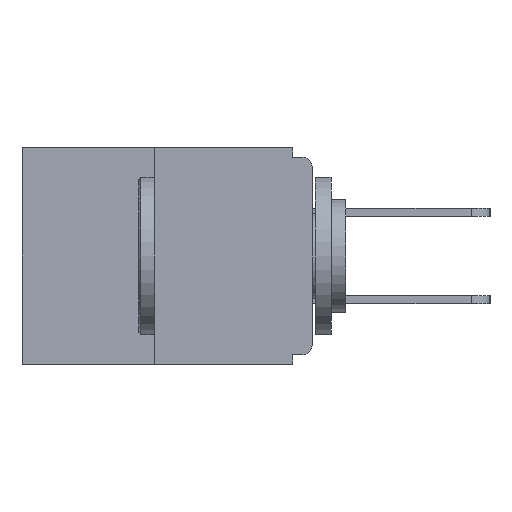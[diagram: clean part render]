
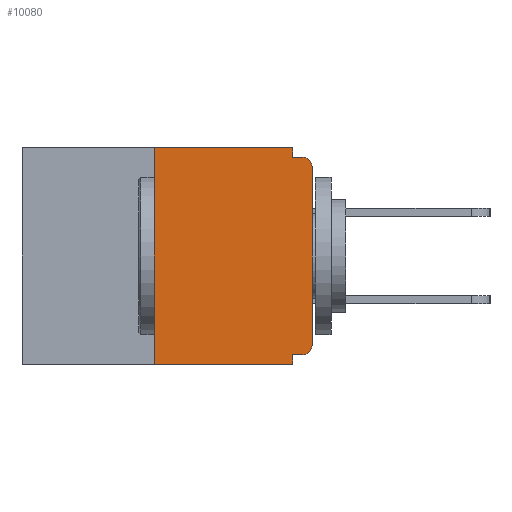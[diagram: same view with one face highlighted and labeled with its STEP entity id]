
A CAD part, left-side view. The second image highlights one B-rep face of the part: STEP entity #10080.
In plain terms, the highlighted planar face has unit normal (-1, 0, 0).
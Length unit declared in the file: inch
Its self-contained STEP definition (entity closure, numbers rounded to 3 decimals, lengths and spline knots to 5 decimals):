
#145 = ORIENTED_EDGE ( 'NONE', *, *, #12287, .T. ) ;
#869 = CARTESIAN_POINT ( 'NONE',  ( 0., 0., -0.03 ) ) ;
#907 = CARTESIAN_POINT ( 'NONE',  ( 0., 0.031, -0.328 ) ) ;
#1152 = CARTESIAN_POINT ( 'NONE',  ( 0., 0.015, -0.313 ) ) ;
#1493 = EDGE_CURVE ( 'NONE', #26048, #3067, #26186, .T. ) ;
#3067 = VERTEX_POINT ( 'NONE', #28551 ) ;
#3303 = ORIENTED_EDGE ( 'NONE', *, *, #7014, .F. ) ;
#3321 = VERTEX_POINT ( 'NONE', #26384 ) ;
#3494 = VERTEX_POINT ( 'NONE', #907 ) ;
#3663 = VECTOR ( 'NONE', #24541, 39.37008 ) ;
#3852 = AXIS2_PLACEMENT_3D ( 'NONE', #1152, #8369, #25537 ) ;
#4375 = CARTESIAN_POINT ( 'NONE',  ( 0., 0., -0.015 ) ) ;
#4817 = LINE ( 'NONE', #4375, #13469 ) ;
#5482 = CARTESIAN_POINT ( 'NONE',  ( 0., 0.46, -0.343 ) ) ;
#6423 = VERTEX_POINT ( 'NONE', #19023 ) ;
#6608 = ORIENTED_EDGE ( 'NONE', *, *, #12519, .F. ) ;
#6713 = VECTOR ( 'NONE', #14352, 39.37008 ) ;
#7014 = EDGE_CURVE ( 'NONE', #6423, #3494, #13935, .T. ) ;
#7239 = LINE ( 'NONE', #16847, #10235 ) ;
#7670 = DIRECTION ( 'NONE',  ( 1., 0., 0. ) ) ;
#8369 = DIRECTION ( 'NONE',  ( -1., 0., 0. ) ) ;
#8530 = LINE ( 'NONE', #5482, #3663 ) ;
#8600 = DIRECTION ( 'NONE',  ( 0., -1., 0. ) ) ;
#8676 = EDGE_CURVE ( 'NONE', #24810, #23961, #8530, .T. ) ;
#8923 = ORIENTED_EDGE ( 'NONE', *, *, #1493, .T. ) ;
#9445 = ORIENTED_EDGE ( 'NONE', *, *, #8676, .T. ) ;
#9480 = EDGE_CURVE ( 'NONE', #3494, #23961, #7239, .T. ) ;
#9860 = DIRECTION ( 'NONE',  ( 0., 0., -1. ) ) ;
#10080 = ADVANCED_FACE ( 'NONE', ( #20475 ), #29157, .F. ) ;
#10235 = VECTOR ( 'NONE', #21683, 39.37008 ) ;
#10701 = CARTESIAN_POINT ( 'NONE',  ( 0., 0., -0.313 ) ) ;
#11185 = EDGE_CURVE ( 'NONE', #29660, #11594, #11668, .T. ) ;
#11594 = VERTEX_POINT ( 'NONE', #20174 ) ;
#11668 = LINE ( 'NONE', #25041, #23734 ) ;
#12287 = EDGE_CURVE ( 'NONE', #6423, #23241, #21100, .T. ) ;
#12415 = CARTESIAN_POINT ( 'NONE',  ( 0., 0.46, 0. ) ) ;
#12519 = EDGE_CURVE ( 'NONE', #11594, #3321, #25159, .T. ) ;
#12708 = DIRECTION ( 'NONE',  ( -1., 0., 0. ) ) ;
#13469 = VECTOR ( 'NONE', #21218, 39.37008 ) ;
#13855 = EDGE_LOOP ( 'NONE', ( #15466, #15655, #9445, #22536, #3303, #145, #29830, #8923, #30356, #6608 ) ) ;
#13935 = LINE ( 'NONE', #28891, #27871 ) ;
#14167 = CARTESIAN_POINT ( 'NONE',  ( 0., 0.031, -0.343 ) ) ;
#14352 = DIRECTION ( 'NONE',  ( 0., 0., -1. ) ) ;
#15230 = DIRECTION ( 'NONE',  ( 0., 0., -1. ) ) ;
#15466 = ORIENTED_EDGE ( 'NONE', *, *, #11185, .F. ) ;
#15655 = ORIENTED_EDGE ( 'NONE', *, *, #23922, .F. ) ;
#15932 = CARTESIAN_POINT ( 'NONE',  ( 0., 0.25, 0. ) ) ;
#16706 = CARTESIAN_POINT ( 'NONE',  ( 0., 0.031, 0. ) ) ;
#16810 = DIRECTION ( 'NONE',  ( 0., 1., 0. ) ) ;
#16847 = CARTESIAN_POINT ( 'NONE',  ( 0., 0.031, -0.343 ) ) ;
#18273 = CARTESIAN_POINT ( 'NONE',  ( 0., 0.25, -0.343 ) ) ;
#19023 = CARTESIAN_POINT ( 'NONE',  ( 0., 0.015, -0.328 ) ) ;
#19800 = EDGE_CURVE ( 'NONE', #3321, #3067, #4817, .T. ) ;
#20174 = CARTESIAN_POINT ( 'NONE',  ( 0., 0.031, 0. ) ) ;
#20475 = FACE_OUTER_BOUND ( 'NONE', #13855, .T. ) ;
#21100 = CIRCLE ( 'NONE', #3852, 0.015 ) ;
#21218 = DIRECTION ( 'NONE',  ( 0., -1., 0. ) ) ;
#21432 = VECTOR ( 'NONE', #28288, 39.37008 ) ;
#21539 = AXIS2_PLACEMENT_3D ( 'NONE', #12415, #7670, #9860 ) ;
#21683 = DIRECTION ( 'NONE',  ( 0., 0., -1. ) ) ;
#22536 = ORIENTED_EDGE ( 'NONE', *, *, #9480, .F. ) ;
#23241 = VERTEX_POINT ( 'NONE', #10701 ) ;
#23441 = CARTESIAN_POINT ( 'NONE',  ( 0., 0., 0. ) ) ;
#23734 = VECTOR ( 'NONE', #8600, 39.37008 ) ;
#23922 = EDGE_CURVE ( 'NONE', #24810, #29660, #26466, .T. ) ;
#23961 = VERTEX_POINT ( 'NONE', #14167 ) ;
#24402 = AXIS2_PLACEMENT_3D ( 'NONE', #24709, #12708, #15230 ) ;
#24541 = DIRECTION ( 'NONE',  ( 0., -1., 0. ) ) ;
#24709 = CARTESIAN_POINT ( 'NONE',  ( 0., 0.015, -0.03 ) ) ;
#24810 = VERTEX_POINT ( 'NONE', #18273 ) ;
#25041 = CARTESIAN_POINT ( 'NONE',  ( 0., 0.46, 0. ) ) ;
#25159 = LINE ( 'NONE', #16706, #6713 ) ;
#25537 = DIRECTION ( 'NONE',  ( 0., 0., -1. ) ) ;
#26048 = VERTEX_POINT ( 'NONE', #869 ) ;
#26079 = DIRECTION ( 'NONE',  ( 0., 0., 1. ) ) ;
#26186 = CIRCLE ( 'NONE', #24402, 0.015 ) ;
#26384 = CARTESIAN_POINT ( 'NONE',  ( 0., 0.031, -0.015 ) ) ;
#26466 = LINE ( 'NONE', #28810, #27981 ) ;
#27072 = LINE ( 'NONE', #23441, #21432 ) ;
#27871 = VECTOR ( 'NONE', #16810, 39.37008 ) ;
#27981 = VECTOR ( 'NONE', #26079, 39.37008 ) ;
#28288 = DIRECTION ( 'NONE',  ( 0., 0., 1. ) ) ;
#28551 = CARTESIAN_POINT ( 'NONE',  ( 0., 0.015, -0.015 ) ) ;
#28810 = CARTESIAN_POINT ( 'NONE',  ( 0., 0.25, 0. ) ) ;
#28891 = CARTESIAN_POINT ( 'NONE',  ( 0., 0., -0.328 ) ) ;
#29157 = PLANE ( 'NONE',  #21539 ) ;
#29660 = VERTEX_POINT ( 'NONE', #15932 ) ;
#29830 = ORIENTED_EDGE ( 'NONE', *, *, #30794, .T. ) ;
#30356 = ORIENTED_EDGE ( 'NONE', *, *, #19800, .F. ) ;
#30794 = EDGE_CURVE ( 'NONE', #23241, #26048, #27072, .T. ) ;
